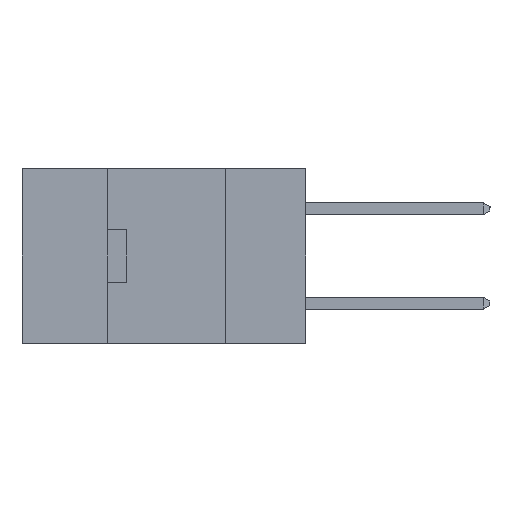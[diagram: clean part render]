
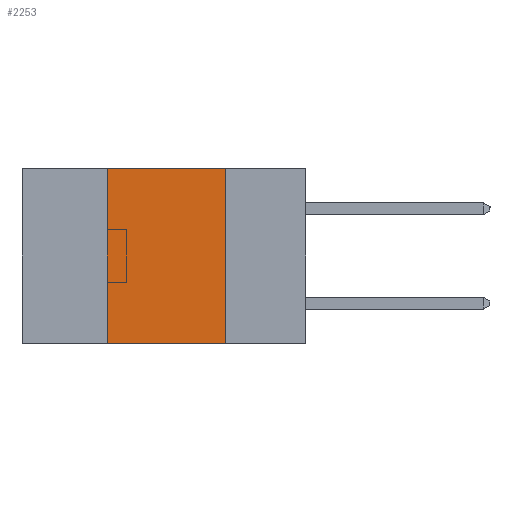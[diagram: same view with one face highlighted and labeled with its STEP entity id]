
A CAD part, left-side view. The second image highlights one B-rep face of the part: STEP entity #2253.
In plain terms, the highlighted planar face has unit normal (-1, 0, 0).
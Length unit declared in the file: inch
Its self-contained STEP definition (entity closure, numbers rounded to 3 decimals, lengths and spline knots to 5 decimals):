
#2146 = VERTEX_POINT ( 'NONE', #17325 ) ;
#2253 = ADVANCED_FACE ( 'NONE', ( #25559 ), #12240, .F. ) ;
#5488 = CARTESIAN_POINT ( 'NONE',  ( 0., 0.42, -0.37 ) ) ;
#5709 = ORIENTED_EDGE ( 'NONE', *, *, #15803, .T. ) ;
#5806 = DIRECTION ( 'NONE',  ( 1., 0., 0. ) ) ;
#7340 = DIRECTION ( 'NONE',  ( 0., -1., 0. ) ) ;
#7884 = CARTESIAN_POINT ( 'NONE',  ( 0., 0.17, -0.37 ) ) ;
#7998 = EDGE_CURVE ( 'NONE', #21577, #2146, #16659, .T. ) ;
#8137 = ORIENTED_EDGE ( 'NONE', *, *, #7998, .F. ) ;
#10233 = VERTEX_POINT ( 'NONE', #5488 ) ;
#11217 = LINE ( 'NONE', #26885, #20888 ) ;
#11585 = LINE ( 'NONE', #25184, #25210 ) ;
#12240 = PLANE ( 'NONE',  #22513 ) ;
#12541 = VERTEX_POINT ( 'NONE', #15244 ) ;
#12713 = EDGE_CURVE ( 'NONE', #10233, #12541, #26821, .T. ) ;
#13555 = DIRECTION ( 'NONE',  ( 0., -1., 0. ) ) ;
#13927 = DIRECTION ( 'NONE',  ( 0., 0., 1. ) ) ;
#15244 = CARTESIAN_POINT ( 'NONE',  ( 0., 0.42, 0. ) ) ;
#15803 = EDGE_CURVE ( 'NONE', #10233, #2146, #11217, .T. ) ;
#16138 = EDGE_LOOP ( 'NONE', ( #8137, #23518, #23801, #5709 ) ) ;
#16659 = LINE ( 'NONE', #7884, #19241 ) ;
#17325 = CARTESIAN_POINT ( 'NONE',  ( 0., 0.17, -0.37 ) ) ;
#18594 = DIRECTION ( 'NONE',  ( 0., 0., -1. ) ) ;
#18706 = DIRECTION ( 'NONE',  ( 0., 0., -1. ) ) ;
#19241 = VECTOR ( 'NONE', #18594, 39.37008 ) ;
#19721 = CARTESIAN_POINT ( 'NONE',  ( 0., 0.17, 0. ) ) ;
#20888 = VECTOR ( 'NONE', #13555, 39.37008 ) ;
#21577 = VERTEX_POINT ( 'NONE', #19721 ) ;
#22283 = CARTESIAN_POINT ( 'NONE',  ( 0., 0.42, -0.37 ) ) ;
#22513 = AXIS2_PLACEMENT_3D ( 'NONE', #28055, #5806, #18706 ) ;
#23518 = ORIENTED_EDGE ( 'NONE', *, *, #28226, .F. ) ;
#23801 = ORIENTED_EDGE ( 'NONE', *, *, #12713, .F. ) ;
#25184 = CARTESIAN_POINT ( 'NONE',  ( 0., 0.6, 0. ) ) ;
#25210 = VECTOR ( 'NONE', #7340, 39.37008 ) ;
#25559 = FACE_OUTER_BOUND ( 'NONE', #16138, .T. ) ;
#26821 = LINE ( 'NONE', #22283, #26830 ) ;
#26830 = VECTOR ( 'NONE', #13927, 39.37008 ) ;
#26885 = CARTESIAN_POINT ( 'NONE',  ( 0., 0.6, -0.37 ) ) ;
#28055 = CARTESIAN_POINT ( 'NONE',  ( 0., 0.6, 0. ) ) ;
#28226 = EDGE_CURVE ( 'NONE', #12541, #21577, #11585, .T. ) ;
